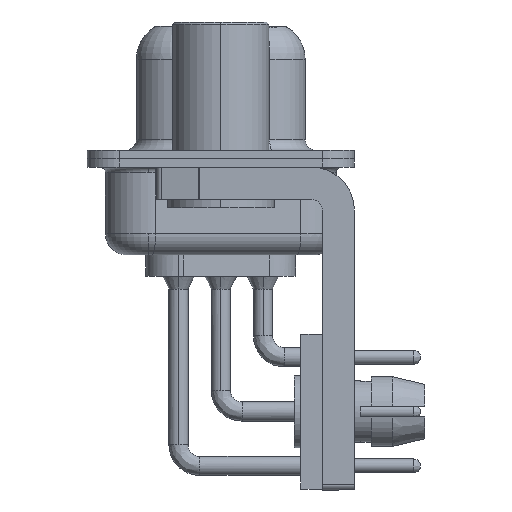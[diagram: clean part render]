
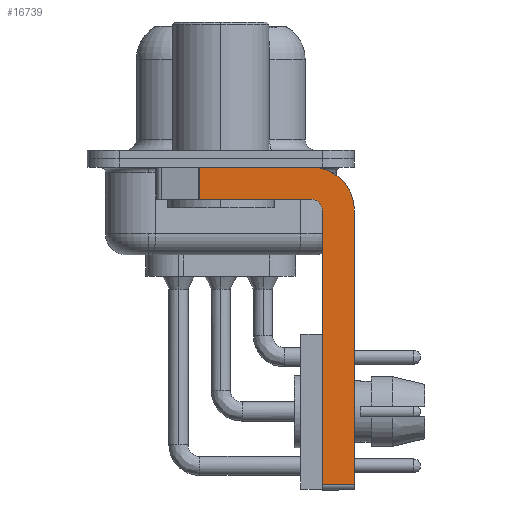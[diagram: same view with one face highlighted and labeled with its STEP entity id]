
A CAD part, left-side view. The second image highlights one B-rep face of the part: STEP entity #16739.
In plain terms, the highlighted planar face has unit normal (-1, 0, 0).
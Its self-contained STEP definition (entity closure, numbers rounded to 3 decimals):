
#51 = CARTESIAN_POINT ( 'NONE',  ( -2.9, 0.978, -1.9 ) ) ;
#512 = DIRECTION ( 'NONE',  ( 0., 0., -1. ) ) ;
#764 = DIRECTION ( 'NONE',  ( -1., 0., 0. ) ) ;
#1130 = VERTEX_POINT ( 'NONE', #18661 ) ;
#2600 = CARTESIAN_POINT ( 'NONE',  ( -2.9, 3., -0.4 ) ) ;
#4073 = EDGE_LOOP ( 'NONE', ( #29103, #27881, #24126, #22416, #25889, #26858, #11250, #7079 ) ) ;
#4252 = DIRECTION ( 'NONE',  ( 0., 1., 0. ) ) ;
#4479 = LINE ( 'NONE', #15702, #21912 ) ;
#4545 = VECTOR ( 'NONE', #20282, 1000. ) ;
#5623 = CARTESIAN_POINT ( 'NONE',  ( -2.9, 0.978, -0.4 ) ) ;
#5686 = AXIS2_PLACEMENT_3D ( 'NONE', #12916, #28935, #15203 ) ;
#6114 = DIRECTION ( 'NONE',  ( 1., 0., 0. ) ) ;
#7079 = ORIENTED_EDGE ( 'NONE', *, *, #29552, .F. ) ;
#7193 = DIRECTION ( 'NONE',  ( 0., -1., 0. ) ) ;
#7312 = EDGE_CURVE ( 'NONE', #18672, #7470, #16152, .T. ) ;
#7338 = EDGE_CURVE ( 'NONE', #18672, #10520, #9383, .T. ) ;
#7470 = VERTEX_POINT ( 'NONE', #25944 ) ;
#8160 = CARTESIAN_POINT ( 'NONE',  ( -2.9, -4.75, -2.4 ) ) ;
#8450 = CARTESIAN_POINT ( 'NONE',  ( -2.9, -6.25, -2.4 ) ) ;
#9383 = LINE ( 'NONE', #9553, #14738 ) ;
#9553 = CARTESIAN_POINT ( 'NONE',  ( -2.9, 0.978, -1.9 ) ) ;
#10520 = VERTEX_POINT ( 'NONE', #51 ) ;
#11024 = VECTOR ( 'NONE', #19568, 1000. ) ;
#11108 = CARTESIAN_POINT ( 'NONE',  ( -2.9, -4.75, -15.25 ) ) ;
#11130 = DIRECTION ( 'NONE',  ( 0., 0., 1. ) ) ;
#11250 = ORIENTED_EDGE ( 'NONE', *, *, #12633, .F. ) ;
#11271 = CARTESIAN_POINT ( 'NONE',  ( -2.9, -6.25, -2.4 ) ) ;
#11738 = LINE ( 'NONE', #28870, #11024 ) ;
#12633 = EDGE_CURVE ( 'NONE', #22385, #1130, #27423, .T. ) ;
#12778 = CARTESIAN_POINT ( 'NONE',  ( -2.9, -4.25, -2.4 ) ) ;
#12916 = CARTESIAN_POINT ( 'NONE',  ( -2.9, -4.25, -2.4 ) ) ;
#14436 = CARTESIAN_POINT ( 'NONE',  ( -2.9, -4.25, -2.4 ) ) ;
#14613 = AXIS2_PLACEMENT_3D ( 'NONE', #12778, #6114, #22030 ) ;
#14738 = VECTOR ( 'NONE', #512, 1000. ) ;
#15058 = VERTEX_POINT ( 'NONE', #11108 ) ;
#15203 = DIRECTION ( 'NONE',  ( 0., 0., -1. ) ) ;
#15702 = CARTESIAN_POINT ( 'NONE',  ( -2.9, -4.25, -1.9 ) ) ;
#16152 = LINE ( 'NONE', #2600, #21479 ) ;
#16670 = DIRECTION ( 'NONE',  ( 0., 0., 1. ) ) ;
#16739 = ADVANCED_FACE ( 'NONE', ( #21373 ), #28906, .F. ) ;
#17390 = VECTOR ( 'NONE', #11130, 1000. ) ;
#17947 = VERTEX_POINT ( 'NONE', #8160 ) ;
#18661 = CARTESIAN_POINT ( 'NONE',  ( -2.9, -6.25, -15.25 ) ) ;
#18672 = VERTEX_POINT ( 'NONE', #5623 ) ;
#19568 = DIRECTION ( 'NONE',  ( 0., -1., 0. ) ) ;
#20282 = DIRECTION ( 'NONE',  ( 0., 0., -1. ) ) ;
#20453 = EDGE_CURVE ( 'NONE', #23317, #10520, #4479, .T. ) ;
#21373 = FACE_OUTER_BOUND ( 'NONE', #4073, .T. ) ;
#21479 = VECTOR ( 'NONE', #7193, 1000. ) ;
#21912 = VECTOR ( 'NONE', #4252, 1000. ) ;
#22030 = DIRECTION ( 'NONE',  ( 0., 0., -1. ) ) ;
#22385 = VERTEX_POINT ( 'NONE', #8450 ) ;
#22416 = ORIENTED_EDGE ( 'NONE', *, *, #27054, .F. ) ;
#22473 = CIRCLE ( 'NONE', #5686, 2. ) ;
#22495 = EDGE_CURVE ( 'NONE', #15058, #17947, #29658, .T. ) ;
#23317 = VERTEX_POINT ( 'NONE', #27786 ) ;
#23640 = EDGE_CURVE ( 'NONE', #15058, #1130, #11738, .T. ) ;
#24126 = ORIENTED_EDGE ( 'NONE', *, *, #20453, .F. ) ;
#25497 = CIRCLE ( 'NONE', #29400, 0.5 ) ;
#25889 = ORIENTED_EDGE ( 'NONE', *, *, #22495, .F. ) ;
#25944 = CARTESIAN_POINT ( 'NONE',  ( -2.9, -4.25, -0.4 ) ) ;
#26858 = ORIENTED_EDGE ( 'NONE', *, *, #23640, .T. ) ;
#27054 = EDGE_CURVE ( 'NONE', #17947, #23317, #25497, .T. ) ;
#27121 = CARTESIAN_POINT ( 'NONE',  ( -2.9, -4.75, -15.5 ) ) ;
#27423 = LINE ( 'NONE', #11271, #4545 ) ;
#27786 = CARTESIAN_POINT ( 'NONE',  ( -2.9, -4.25, -1.9 ) ) ;
#27881 = ORIENTED_EDGE ( 'NONE', *, *, #7338, .T. ) ;
#28870 = CARTESIAN_POINT ( 'NONE',  ( -2.9, -4.25, -15.25 ) ) ;
#28906 = PLANE ( 'NONE',  #14613 ) ;
#28935 = DIRECTION ( 'NONE',  ( 1., 0., 0. ) ) ;
#29103 = ORIENTED_EDGE ( 'NONE', *, *, #7312, .F. ) ;
#29400 = AXIS2_PLACEMENT_3D ( 'NONE', #14436, #764, #16670 ) ;
#29552 = EDGE_CURVE ( 'NONE', #7470, #22385, #22473, .T. ) ;
#29658 = LINE ( 'NONE', #27121, #17390 ) ;
